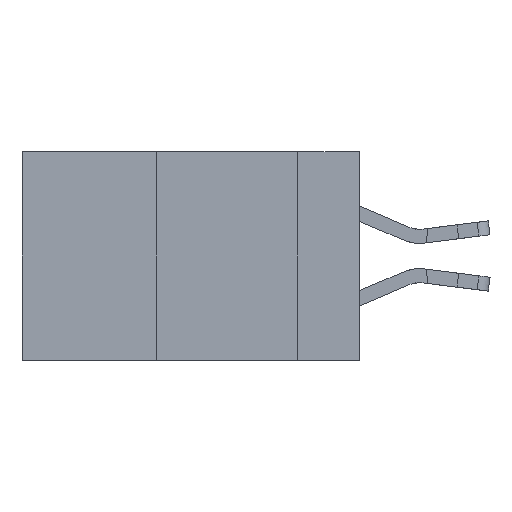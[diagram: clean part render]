
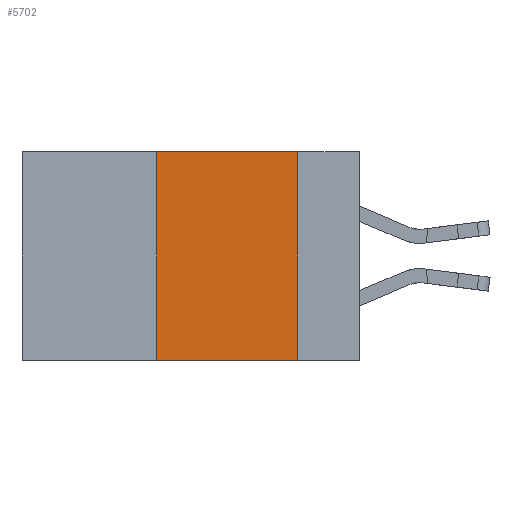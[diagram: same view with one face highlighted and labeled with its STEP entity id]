
A CAD part, left-side view. The second image highlights one B-rep face of the part: STEP entity #5702.
In plain terms, the highlighted planar face has unit normal (-1, 0, 0).
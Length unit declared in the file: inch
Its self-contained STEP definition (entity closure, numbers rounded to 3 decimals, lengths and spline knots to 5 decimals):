
#254 = VECTOR ( 'NONE', #12203, 39.37008 ) ;
#297 = LINE ( 'NONE', #12701, #8737 ) ;
#528 = CARTESIAN_POINT ( 'NONE',  ( 0., 0.36, -0.37 ) ) ;
#1490 = DIRECTION ( 'NONE',  ( 0., 0., 1. ) ) ;
#2112 = LINE ( 'NONE', #14302, #254 ) ;
#2164 = DIRECTION ( 'NONE',  ( 0., -1., 0. ) ) ;
#2695 = DIRECTION ( 'NONE',  ( 0., 0., -1. ) ) ;
#2938 = CARTESIAN_POINT ( 'NONE',  ( 0., 0.11, -0.37 ) ) ;
#2959 = DIRECTION ( 'NONE',  ( 1., 0., 0. ) ) ;
#3083 = CARTESIAN_POINT ( 'NONE',  ( 0., 0.6, 0. ) ) ;
#4174 = EDGE_CURVE ( 'NONE', #9971, #13727, #297, .T. ) ;
#5583 = FACE_OUTER_BOUND ( 'NONE', #8772, .T. ) ;
#5702 = ADVANCED_FACE ( 'NONE', ( #5583 ), #14819, .F. ) ;
#6159 = ORIENTED_EDGE ( 'NONE', *, *, #9977, .F. ) ;
#6243 = ORIENTED_EDGE ( 'NONE', *, *, #12662, .T. ) ;
#6391 = EDGE_CURVE ( 'NONE', #7226, #11704, #12563, .T. ) ;
#7226 = VERTEX_POINT ( 'NONE', #528 ) ;
#8737 = VECTOR ( 'NONE', #2695, 39.37008 ) ;
#8772 = EDGE_LOOP ( 'NONE', ( #13884, #6159, #12773, #6243 ) ) ;
#9897 = VECTOR ( 'NONE', #1490, 39.37008 ) ;
#9971 = VERTEX_POINT ( 'NONE', #13142 ) ;
#9977 = EDGE_CURVE ( 'NONE', #11704, #9971, #2112, .T. ) ;
#11704 = VERTEX_POINT ( 'NONE', #12211 ) ;
#12109 = VECTOR ( 'NONE', #2164, 39.37008 ) ;
#12203 = DIRECTION ( 'NONE',  ( 0., -1., 0. ) ) ;
#12211 = CARTESIAN_POINT ( 'NONE',  ( 0., 0.36, 0. ) ) ;
#12282 = DIRECTION ( 'NONE',  ( 0., 0., -1. ) ) ;
#12563 = LINE ( 'NONE', #15961, #9897 ) ;
#12662 = EDGE_CURVE ( 'NONE', #7226, #13727, #15599, .T. ) ;
#12701 = CARTESIAN_POINT ( 'NONE',  ( 0., 0.11, 0. ) ) ;
#12773 = ORIENTED_EDGE ( 'NONE', *, *, #6391, .F. ) ;
#13142 = CARTESIAN_POINT ( 'NONE',  ( 0., 0.11, 0. ) ) ;
#13727 = VERTEX_POINT ( 'NONE', #2938 ) ;
#13752 = AXIS2_PLACEMENT_3D ( 'NONE', #3083, #2959, #12282 ) ;
#13884 = ORIENTED_EDGE ( 'NONE', *, *, #4174, .F. ) ;
#14302 = CARTESIAN_POINT ( 'NONE',  ( 0., 0.6, 0. ) ) ;
#14819 = PLANE ( 'NONE',  #13752 ) ;
#15599 = LINE ( 'NONE', #16802, #12109 ) ;
#15961 = CARTESIAN_POINT ( 'NONE',  ( 0., 0.36, 0. ) ) ;
#16802 = CARTESIAN_POINT ( 'NONE',  ( 0., 0.6, -0.37 ) ) ;
